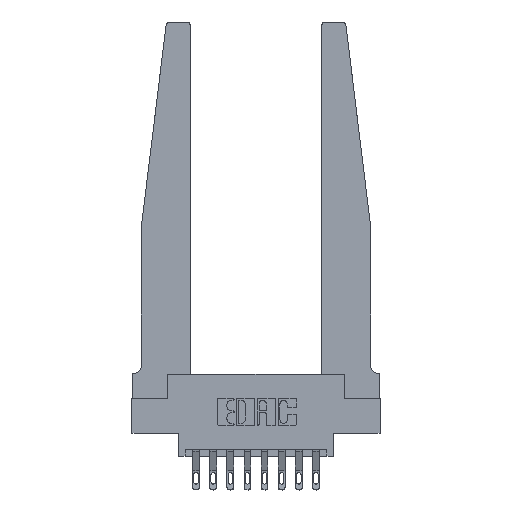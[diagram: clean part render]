
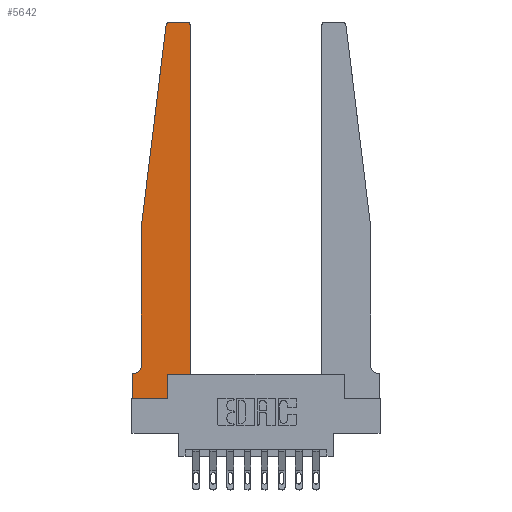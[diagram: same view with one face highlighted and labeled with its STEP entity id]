
A CAD part, top view. The second image highlights one B-rep face of the part: STEP entity #5642.
In plain terms, the highlighted planar face has unit normal (0, 0, 1).
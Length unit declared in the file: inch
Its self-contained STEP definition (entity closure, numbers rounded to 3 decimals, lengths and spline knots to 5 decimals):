
#178 = VERTEX_POINT ( 'NONE', #8035 ) ;
#547 = CARTESIAN_POINT ( 'NONE',  ( 0.24675, 2.72367, 0.37 ) ) ;
#991 = LINE ( 'NONE', #13094, #1879 ) ;
#1050 = VECTOR ( 'NONE', #9127, 39.37008 ) ;
#1204 = EDGE_CURVE ( 'NONE', #7164, #8944, #4839, .T. ) ;
#1232 = DIRECTION ( 'NONE',  ( 0., -1., 0. ) ) ;
#1398 = CARTESIAN_POINT ( 'NONE',  ( 0.425, 2.72, 0.37 ) ) ;
#1451 = EDGE_CURVE ( 'NONE', #5675, #12337, #991, .T. ) ;
#1478 = DIRECTION ( 'NONE',  ( -1., 0., 0. ) ) ;
#1491 = AXIS2_PLACEMENT_3D ( 'NONE', #4071, #10050, #6409 ) ;
#1518 = CIRCLE ( 'NONE', #14784, 0.03 ) ;
#1575 = DIRECTION ( 'NONE',  ( -1., 0., 0. ) ) ;
#1590 = ORIENTED_EDGE ( 'NONE', *, *, #3040, .T. ) ;
#1684 = LINE ( 'NONE', #4479, #4808 ) ;
#1879 = VECTOR ( 'NONE', #14285, 39.37008 ) ;
#2079 = CARTESIAN_POINT ( 'NONE',  ( 0.065, 0.1875, 0.37 ) ) ;
#2313 = CIRCLE ( 'NONE', #6585, 0.03 ) ;
#2407 = ORIENTED_EDGE ( 'NONE', *, *, #11867, .T. ) ;
#2478 = CARTESIAN_POINT ( 'NONE',  ( 0., 0., 0.37 ) ) ;
#2701 = CARTESIAN_POINT ( 'NONE',  ( 0.2605, 0.18, 0.37 ) ) ;
#2716 = ORIENTED_EDGE ( 'NONE', *, *, #1204, .T. ) ;
#2752 = DIRECTION ( 'NONE',  ( 1., 0., 0. ) ) ;
#2781 = ORIENTED_EDGE ( 'NONE', *, *, #8285, .T. ) ;
#3040 = EDGE_CURVE ( 'NONE', #4048, #11241, #3247, .T. ) ;
#3246 = CARTESIAN_POINT ( 'NONE',  ( 0.065, 0.2375, 0.37 ) ) ;
#3247 = LINE ( 'NONE', #2079, #10837 ) ;
#3505 = CARTESIAN_POINT ( 'NONE',  ( 0.065, 1.25, 0.37 ) ) ;
#3567 = CARTESIAN_POINT ( 'NONE',  ( 0., 0.1875, 0.37 ) ) ;
#3672 = DIRECTION ( 'NONE',  ( 0., 0., 1. ) ) ;
#3848 = ORIENTED_EDGE ( 'NONE', *, *, #12184, .T. ) ;
#3869 = CARTESIAN_POINT ( 'NONE',  ( 0.27653, 2.72, 0.37 ) ) ;
#3899 = CARTESIAN_POINT ( 'NONE',  ( 0.2605, 0.18, 0.37 ) ) ;
#4048 = VERTEX_POINT ( 'NONE', #5245 ) ;
#4071 = CARTESIAN_POINT ( 'NONE',  ( 0., 0.1875, 0.37 ) ) ;
#4400 = CARTESIAN_POINT ( 'NONE',  ( 0.425, 0.18, 0.37 ) ) ;
#4479 = CARTESIAN_POINT ( 'NONE',  ( 0., 0., 0.37 ) ) ;
#4514 = DIRECTION ( 'NONE',  ( -1., 0., 0. ) ) ;
#4783 = ORIENTED_EDGE ( 'NONE', *, *, #10898, .T. ) ;
#4808 = VECTOR ( 'NONE', #9212, 39.37008 ) ;
#4839 = LINE ( 'NONE', #3899, #7348 ) ;
#4857 = LINE ( 'NONE', #2478, #6984 ) ;
#5245 = CARTESIAN_POINT ( 'NONE',  ( 0.015, 0.1875, 0.37 ) ) ;
#5312 = FACE_OUTER_BOUND ( 'NONE', #11906, .T. ) ;
#5514 = EDGE_CURVE ( 'NONE', #6230, #7164, #4857, .T. ) ;
#5642 = ADVANCED_FACE ( 'NONE', ( #5312 ), #11221, .T. ) ;
#5675 = VERTEX_POINT ( 'NONE', #547 ) ;
#5771 = ORIENTED_EDGE ( 'NONE', *, *, #12376, .T. ) ;
#6191 = CARTESIAN_POINT ( 'NONE',  ( 0.015, 0.2375, 0.37 ) ) ;
#6230 = VERTEX_POINT ( 'NONE', #12276 ) ;
#6409 = DIRECTION ( 'NONE',  ( 1., 0., 0. ) ) ;
#6550 = CIRCLE ( 'NONE', #9766, 0.05 ) ;
#6585 = AXIS2_PLACEMENT_3D ( 'NONE', #10526, #3672, #12882 ) ;
#6626 = DIRECTION ( 'NONE',  ( 0., 1., 0. ) ) ;
#6984 = VECTOR ( 'NONE', #11856, 39.37008 ) ;
#7164 = VERTEX_POINT ( 'NONE', #7327 ) ;
#7327 = CARTESIAN_POINT ( 'NONE',  ( 0.2605, 0., 0.37 ) ) ;
#7348 = VECTOR ( 'NONE', #13342, 39.37008 ) ;
#7632 = LINE ( 'NONE', #10020, #8278 ) ;
#7636 = ORIENTED_EDGE ( 'NONE', *, *, #7765, .T. ) ;
#7710 = EDGE_CURVE ( 'NONE', #8777, #8506, #7632, .T. ) ;
#7765 = EDGE_CURVE ( 'NONE', #11241, #6230, #1684, .T. ) ;
#8035 = CARTESIAN_POINT ( 'NONE',  ( 0.395, 2.75, 0.37 ) ) ;
#8278 = VECTOR ( 'NONE', #6626, 39.37008 ) ;
#8285 = EDGE_CURVE ( 'NONE', #12337, #11197, #10512, .T. ) ;
#8339 = VECTOR ( 'NONE', #1575, 39.37008 ) ;
#8506 = VERTEX_POINT ( 'NONE', #1398 ) ;
#8687 = DIRECTION ( 'NONE',  ( 0., 0., 1. ) ) ;
#8777 = VERTEX_POINT ( 'NONE', #9415 ) ;
#8944 = VERTEX_POINT ( 'NONE', #2701 ) ;
#9127 = DIRECTION ( 'NONE',  ( 1., 0., 0. ) ) ;
#9212 = DIRECTION ( 'NONE',  ( 0., -1., 0. ) ) ;
#9415 = CARTESIAN_POINT ( 'NONE',  ( 0.425, 0.18, 0.37 ) ) ;
#9497 = ORIENTED_EDGE ( 'NONE', *, *, #1451, .T. ) ;
#9621 = CARTESIAN_POINT ( 'NONE',  ( 0.25, 2.75, 0.37 ) ) ;
#9736 = ORIENTED_EDGE ( 'NONE', *, *, #10612, .T. ) ;
#9766 = AXIS2_PLACEMENT_3D ( 'NONE', #6191, #13373, #1478 ) ;
#9913 = VERTEX_POINT ( 'NONE', #15401 ) ;
#10020 = CARTESIAN_POINT ( 'NONE',  ( 0.425, 0.18, 0.37 ) ) ;
#10050 = DIRECTION ( 'NONE',  ( 0., 0., 1. ) ) ;
#10512 = LINE ( 'NONE', #3505, #15293 ) ;
#10526 = CARTESIAN_POINT ( 'NONE',  ( 0.395, 2.72, 0.37 ) ) ;
#10612 = EDGE_CURVE ( 'NONE', #178, #9913, #12117, .T. ) ;
#10837 = VECTOR ( 'NONE', #4514, 39.37008 ) ;
#10898 = EDGE_CURVE ( 'NONE', #8506, #178, #2313, .T. ) ;
#11197 = VERTEX_POINT ( 'NONE', #3246 ) ;
#11214 = ORIENTED_EDGE ( 'NONE', *, *, #7710, .T. ) ;
#11221 = PLANE ( 'NONE',  #1491 ) ;
#11241 = VERTEX_POINT ( 'NONE', #3567 ) ;
#11856 = DIRECTION ( 'NONE',  ( 1., 0., 0. ) ) ;
#11867 = EDGE_CURVE ( 'NONE', #9913, #5675, #1518, .T. ) ;
#11906 = EDGE_LOOP ( 'NONE', ( #9736, #2407, #9497, #2781, #3848, #1590, #7636, #14031, #2716, #5771, #11214, #4783 ) ) ;
#12117 = LINE ( 'NONE', #9621, #8339 ) ;
#12184 = EDGE_CURVE ( 'NONE', #11197, #4048, #6550, .T. ) ;
#12276 = CARTESIAN_POINT ( 'NONE',  ( 0., 0., 0.37 ) ) ;
#12337 = VERTEX_POINT ( 'NONE', #14956 ) ;
#12344 = LINE ( 'NONE', #4400, #1050 ) ;
#12376 = EDGE_CURVE ( 'NONE', #8944, #8777, #12344, .T. ) ;
#12882 = DIRECTION ( 'NONE',  ( 1., 0., 0. ) ) ;
#13094 = CARTESIAN_POINT ( 'NONE',  ( 0.065, 1.25, 0.37 ) ) ;
#13342 = DIRECTION ( 'NONE',  ( 0., 1., 0. ) ) ;
#13373 = DIRECTION ( 'NONE',  ( 0., 0., -1. ) ) ;
#14031 = ORIENTED_EDGE ( 'NONE', *, *, #5514, .T. ) ;
#14285 = DIRECTION ( 'NONE',  ( -0.122, -0.992, 0. ) ) ;
#14784 = AXIS2_PLACEMENT_3D ( 'NONE', #3869, #8687, #2752 ) ;
#14956 = CARTESIAN_POINT ( 'NONE',  ( 0.065, 1.25, 0.37 ) ) ;
#15293 = VECTOR ( 'NONE', #1232, 39.37008 ) ;
#15401 = CARTESIAN_POINT ( 'NONE',  ( 0.27653, 2.75, 0.37 ) ) ;
